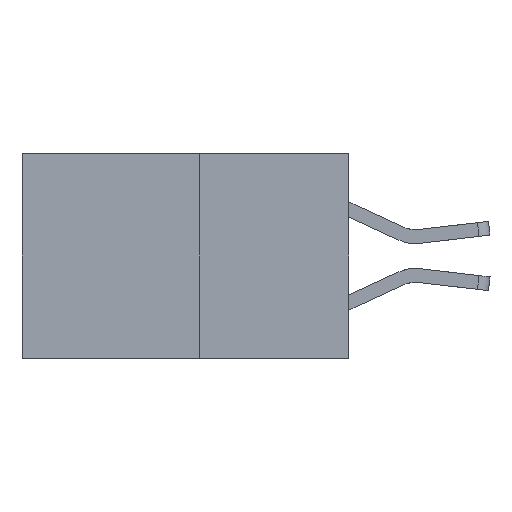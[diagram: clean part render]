
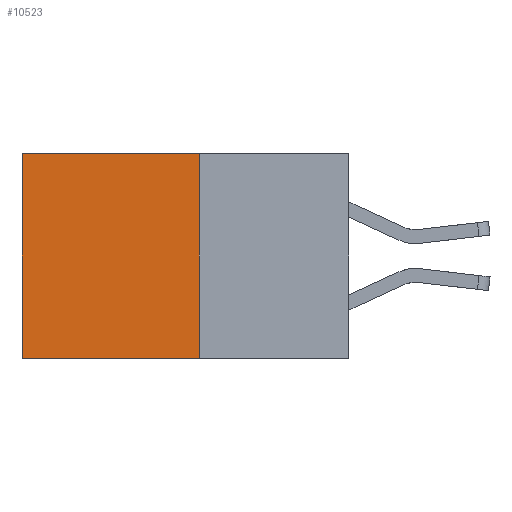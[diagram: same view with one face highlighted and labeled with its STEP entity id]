
A CAD part, left-side view. The second image highlights one B-rep face of the part: STEP entity #10523.
In plain terms, the highlighted planar face has unit normal (-1, 0, 0).
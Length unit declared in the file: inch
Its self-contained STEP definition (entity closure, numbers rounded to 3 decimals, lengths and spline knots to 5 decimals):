
#29 = LINE ( 'NONE', #10780, #4438 ) ;
#168 = CARTESIAN_POINT ( 'NONE',  ( 0.277, 0.59, 0. ) ) ;
#171 = LINE ( 'NONE', #9965, #9232 ) ;
#597 = PLANE ( 'NONE',  #10065 ) ;
#1552 = CARTESIAN_POINT ( 'NONE',  ( 0.277, 0.27, -0.37 ) ) ;
#2406 = VERTEX_POINT ( 'NONE', #6149 ) ;
#2412 = DIRECTION ( 'NONE',  ( 0., 0., -1. ) ) ;
#2457 = EDGE_CURVE ( 'NONE', #6636, #8875, #5468, .T. ) ;
#3264 = DIRECTION ( 'NONE',  ( 0., 0., -1. ) ) ;
#4379 = LINE ( 'NONE', #10015, #6131 ) ;
#4438 = VECTOR ( 'NONE', #3264, 39.37008 ) ;
#4844 = ORIENTED_EDGE ( 'NONE', *, *, #5919, .T. ) ;
#5281 = ORIENTED_EDGE ( 'NONE', *, *, #8294, .F. ) ;
#5468 = LINE ( 'NONE', #11102, #7528 ) ;
#5554 = DIRECTION ( 'NONE',  ( 0., 0., -1. ) ) ;
#5659 = EDGE_CURVE ( 'NONE', #6636, #9144, #171, .T. ) ;
#5919 = EDGE_CURVE ( 'NONE', #8875, #2406, #29, .T. ) ;
#6131 = VECTOR ( 'NONE', #7950, 39.37008 ) ;
#6149 = CARTESIAN_POINT ( 'NONE',  ( 0.277, 0.59, -0.37 ) ) ;
#6636 = VERTEX_POINT ( 'NONE', #9522 ) ;
#6697 = CARTESIAN_POINT ( 'NONE',  ( 0.277, 0.27, -0.37 ) ) ;
#7528 = VECTOR ( 'NONE', #10715, 39.37008 ) ;
#7605 = FACE_OUTER_BOUND ( 'NONE', #7918, .T. ) ;
#7650 = DIRECTION ( 'NONE',  ( 1., 0., 0. ) ) ;
#7918 = EDGE_LOOP ( 'NONE', ( #4844, #5281, #9799, #8029 ) ) ;
#7950 = DIRECTION ( 'NONE',  ( 0., 1., 0. ) ) ;
#8029 = ORIENTED_EDGE ( 'NONE', *, *, #2457, .T. ) ;
#8294 = EDGE_CURVE ( 'NONE', #9144, #2406, #4379, .T. ) ;
#8875 = VERTEX_POINT ( 'NONE', #168 ) ;
#9144 = VERTEX_POINT ( 'NONE', #6697 ) ;
#9232 = VECTOR ( 'NONE', #5554, 39.37008 ) ;
#9522 = CARTESIAN_POINT ( 'NONE',  ( 0.277, 0.27, 0. ) ) ;
#9799 = ORIENTED_EDGE ( 'NONE', *, *, #5659, .F. ) ;
#9965 = CARTESIAN_POINT ( 'NONE',  ( 0.277, 0.27, -0.37 ) ) ;
#10015 = CARTESIAN_POINT ( 'NONE',  ( 0.277, 0.27, -0.37 ) ) ;
#10065 = AXIS2_PLACEMENT_3D ( 'NONE', #1552, #7650, #2412 ) ;
#10523 = ADVANCED_FACE ( 'NONE', ( #7605 ), #597, .F. ) ;
#10715 = DIRECTION ( 'NONE',  ( 0., 1., 0. ) ) ;
#10780 = CARTESIAN_POINT ( 'NONE',  ( 0.277, 0.59, -0.37 ) ) ;
#11102 = CARTESIAN_POINT ( 'NONE',  ( 0.277, 0.27, 0. ) ) ;
